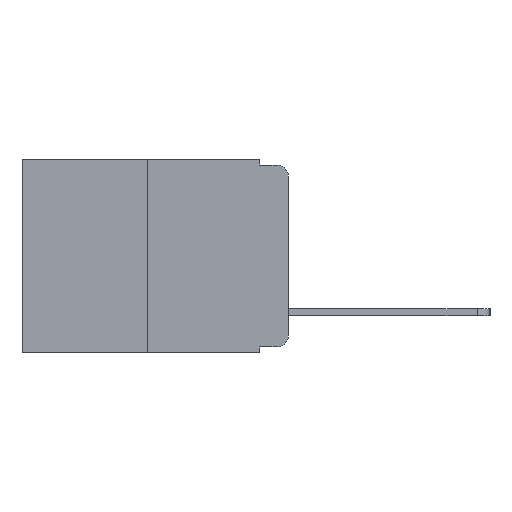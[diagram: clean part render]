
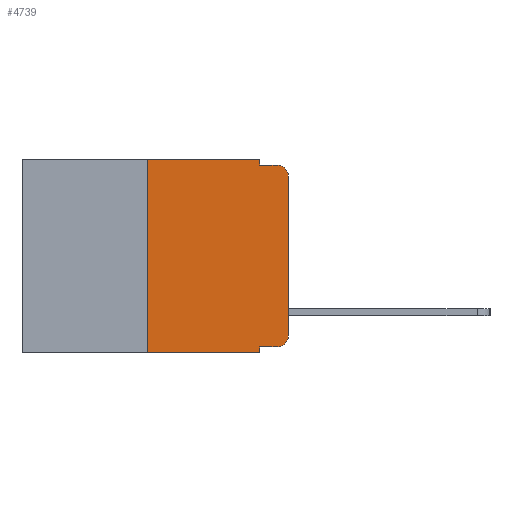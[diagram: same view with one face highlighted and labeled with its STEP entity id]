
A CAD part, left-side view. The second image highlights one B-rep face of the part: STEP entity #4739.
In plain terms, the highlighted planar face has unit normal (-1, 0, 0).
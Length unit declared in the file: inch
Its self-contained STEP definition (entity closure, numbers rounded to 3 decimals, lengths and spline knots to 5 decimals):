
#23 = ORIENTED_EDGE ( 'NONE', *, *, #21287, .T. ) ;
#149 = EDGE_CURVE ( 'NONE', #20082, #487, #14431, .T. ) ;
#487 = VERTEX_POINT ( 'NONE', #23990 ) ;
#1047 = CARTESIAN_POINT ( 'NONE',  ( 0., 0.25, 0. ) ) ;
#1213 = LINE ( 'NONE', #13328, #10876 ) ;
#1237 = CARTESIAN_POINT ( 'NONE',  ( 0., 0.02, -0.313 ) ) ;
#1860 = ORIENTED_EDGE ( 'NONE', *, *, #16153, .F. ) ;
#2201 = CARTESIAN_POINT ( 'NONE',  ( 0., 0.473, 0. ) ) ;
#2288 = AXIS2_PLACEMENT_3D ( 'NONE', #6942, #20243, #8854 ) ;
#2344 = VERTEX_POINT ( 'NONE', #19228 ) ;
#2377 = VERTEX_POINT ( 'NONE', #16392 ) ;
#2487 = EDGE_LOOP ( 'NONE', ( #23, #22510, #10726, #1860, #20133, #16595, #13057, #12153, #15412, #8848 ) ) ;
#3105 = EDGE_CURVE ( 'NONE', #19577, #2344, #6208, .T. ) ;
#3220 = DIRECTION ( 'NONE',  ( 0., 0., -1. ) ) ;
#3247 = DIRECTION ( 'NONE',  ( 0., 0., -1. ) ) ;
#3855 = VERTEX_POINT ( 'NONE', #6285 ) ;
#4562 = EDGE_CURVE ( 'NONE', #2377, #24487, #18108, .T. ) ;
#4739 = ADVANCED_FACE ( 'NONE', ( #23306 ), #18600, .F. ) ;
#5519 = EDGE_CURVE ( 'NONE', #2377, #22405, #7292, .T. ) ;
#5970 = CARTESIAN_POINT ( 'NONE',  ( 0., 0., -0.03 ) ) ;
#6208 = LINE ( 'NONE', #22486, #12494 ) ;
#6285 = CARTESIAN_POINT ( 'NONE',  ( 0., 0.051, 0. ) ) ;
#6328 = CARTESIAN_POINT ( 'NONE',  ( 0., 0.051, -0.333 ) ) ;
#6942 = CARTESIAN_POINT ( 'NONE',  ( 0., 0.02, -0.03 ) ) ;
#7017 = CARTESIAN_POINT ( 'NONE',  ( 0., 0.051, 0. ) ) ;
#7292 = LINE ( 'NONE', #7938, #13617 ) ;
#7938 = CARTESIAN_POINT ( 'NONE',  ( 0., 0.473, -0.343 ) ) ;
#7940 = VECTOR ( 'NONE', #12658, 39.37008 ) ;
#7961 = AXIS2_PLACEMENT_3D ( 'NONE', #2201, #16872, #3247 ) ;
#8037 = LINE ( 'NONE', #8719, #13144 ) ;
#8305 = EDGE_CURVE ( 'NONE', #24487, #3855, #23920, .T. ) ;
#8614 = CIRCLE ( 'NONE', #2288, 0.02 ) ;
#8719 = CARTESIAN_POINT ( 'NONE',  ( 0., 0., 0. ) ) ;
#8848 = ORIENTED_EDGE ( 'NONE', *, *, #15971, .T. ) ;
#8854 = DIRECTION ( 'NONE',  ( 0., 0., -1. ) ) ;
#8859 = CARTESIAN_POINT ( 'NONE',  ( 0., 0.051, -0.333 ) ) ;
#8878 = CARTESIAN_POINT ( 'NONE',  ( 0., 0.051, -0.343 ) ) ;
#9498 = DIRECTION ( 'NONE',  ( 0., -1., 0. ) ) ;
#9994 = CIRCLE ( 'NONE', #22585, 0.02 ) ;
#10726 = ORIENTED_EDGE ( 'NONE', *, *, #3105, .F. ) ;
#10768 = VERTEX_POINT ( 'NONE', #13081 ) ;
#10876 = VECTOR ( 'NONE', #22771, 39.37008 ) ;
#11167 = DIRECTION ( 'NONE',  ( 0., -1., 0. ) ) ;
#11699 = DIRECTION ( 'NONE',  ( 0., -1., 0. ) ) ;
#12153 = ORIENTED_EDGE ( 'NONE', *, *, #23004, .F. ) ;
#12494 = VECTOR ( 'NONE', #9498, 39.37008 ) ;
#12658 = DIRECTION ( 'NONE',  ( 0., 0., 1. ) ) ;
#13057 = ORIENTED_EDGE ( 'NONE', *, *, #5519, .T. ) ;
#13081 = CARTESIAN_POINT ( 'NONE',  ( 0., 0., -0.313 ) ) ;
#13144 = VECTOR ( 'NONE', #20190, 39.37008 ) ;
#13328 = CARTESIAN_POINT ( 'NONE',  ( 0., 0.051, 0. ) ) ;
#13617 = VECTOR ( 'NONE', #11699, 39.37008 ) ;
#14000 = VECTOR ( 'NONE', #18452, 39.37008 ) ;
#14012 = CARTESIAN_POINT ( 'NONE',  ( 0., 0.25, 0. ) ) ;
#14431 = LINE ( 'NONE', #6328, #23780 ) ;
#14718 = CARTESIAN_POINT ( 'NONE',  ( 0., 0.473, 0. ) ) ;
#14772 = DIRECTION ( 'NONE',  ( -1., 0., 0. ) ) ;
#15412 = ORIENTED_EDGE ( 'NONE', *, *, #149, .T. ) ;
#15971 = EDGE_CURVE ( 'NONE', #487, #10768, #9994, .T. ) ;
#16153 = EDGE_CURVE ( 'NONE', #3855, #19577, #1213, .T. ) ;
#16392 = CARTESIAN_POINT ( 'NONE',  ( 0., 0.25, -0.343 ) ) ;
#16595 = ORIENTED_EDGE ( 'NONE', *, *, #4562, .F. ) ;
#16872 = DIRECTION ( 'NONE',  ( 1., 0., 0. ) ) ;
#17718 = VERTEX_POINT ( 'NONE', #5970 ) ;
#18108 = LINE ( 'NONE', #1047, #7940 ) ;
#18452 = DIRECTION ( 'NONE',  ( 0., 0., -1. ) ) ;
#18600 = PLANE ( 'NONE',  #7961 ) ;
#19019 = VECTOR ( 'NONE', #22155, 39.37008 ) ;
#19228 = CARTESIAN_POINT ( 'NONE',  ( 0., 0.02, -0.01 ) ) ;
#19577 = VERTEX_POINT ( 'NONE', #22143 ) ;
#20082 = VERTEX_POINT ( 'NONE', #8859 ) ;
#20133 = ORIENTED_EDGE ( 'NONE', *, *, #8305, .F. ) ;
#20190 = DIRECTION ( 'NONE',  ( 0., 0., 1. ) ) ;
#20243 = DIRECTION ( 'NONE',  ( -1., 0., 0. ) ) ;
#21287 = EDGE_CURVE ( 'NONE', #10768, #17718, #8037, .T. ) ;
#21931 = EDGE_CURVE ( 'NONE', #17718, #2344, #8614, .T. ) ;
#22143 = CARTESIAN_POINT ( 'NONE',  ( 0., 0.051, -0.01 ) ) ;
#22155 = DIRECTION ( 'NONE',  ( 0., -1., 0. ) ) ;
#22405 = VERTEX_POINT ( 'NONE', #8878 ) ;
#22486 = CARTESIAN_POINT ( 'NONE',  ( 0., 0.051, -0.01 ) ) ;
#22510 = ORIENTED_EDGE ( 'NONE', *, *, #21931, .T. ) ;
#22585 = AXIS2_PLACEMENT_3D ( 'NONE', #1237, #14772, #3220 ) ;
#22771 = DIRECTION ( 'NONE',  ( 0., 0., -1. ) ) ;
#22796 = LINE ( 'NONE', #7017, #14000 ) ;
#23004 = EDGE_CURVE ( 'NONE', #20082, #22405, #22796, .T. ) ;
#23306 = FACE_OUTER_BOUND ( 'NONE', #2487, .T. ) ;
#23780 = VECTOR ( 'NONE', #11167, 39.37008 ) ;
#23920 = LINE ( 'NONE', #14718, #19019 ) ;
#23990 = CARTESIAN_POINT ( 'NONE',  ( 0., 0.02, -0.333 ) ) ;
#24487 = VERTEX_POINT ( 'NONE', #14012 ) ;
